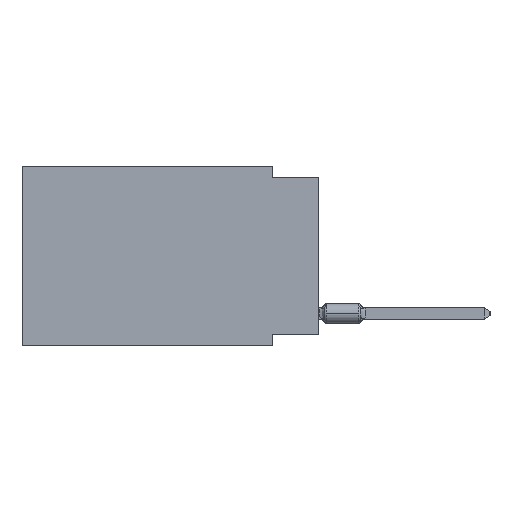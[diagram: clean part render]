
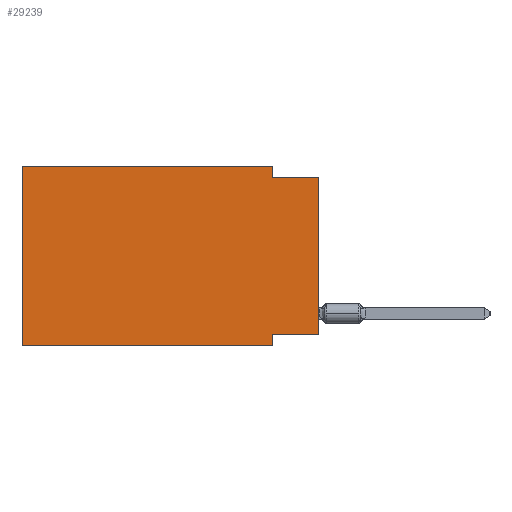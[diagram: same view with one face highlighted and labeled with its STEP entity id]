
A CAD part, left-side view. The second image highlights one B-rep face of the part: STEP entity #29239.
In plain terms, the highlighted planar face has unit normal (-1, 0, 0).
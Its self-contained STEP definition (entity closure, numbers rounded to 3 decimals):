
#490 = VECTOR ( 'NONE', #22707, 1000. ) ;
#543 = DIRECTION ( 'NONE',  ( 0., 0., 1. ) ) ;
#1589 = ORIENTED_EDGE ( 'NONE', *, *, #5395, .T. ) ;
#1787 = LINE ( 'NONE', #32065, #10415 ) ;
#1984 = CARTESIAN_POINT ( 'NONE',  ( 0., 0., -0.635 ) ) ;
#2835 = CARTESIAN_POINT ( 'NONE',  ( 0., 2.54, 0. ) ) ;
#3249 = CARTESIAN_POINT ( 'NONE',  ( 0., 2.54, -9.906 ) ) ;
#4704 = DIRECTION ( 'NONE',  ( 0., -1., 0. ) ) ;
#5305 = CARTESIAN_POINT ( 'NONE',  ( 0., 16.383, 0. ) ) ;
#5395 = EDGE_CURVE ( 'NONE', #22550, #21201, #22999, .T. ) ;
#6250 = LINE ( 'NONE', #11909, #23976 ) ;
#6570 = CARTESIAN_POINT ( 'NONE',  ( 0., 2.54, -9.906 ) ) ;
#6589 = VECTOR ( 'NONE', #13106, 1000. ) ;
#8101 = AXIS2_PLACEMENT_3D ( 'NONE', #5305, #10420, #24469 ) ;
#8115 = DIRECTION ( 'NONE',  ( 0., 1., 0. ) ) ;
#8686 = VERTEX_POINT ( 'NONE', #35474 ) ;
#9042 = VERTEX_POINT ( 'NONE', #18314 ) ;
#10415 = VECTOR ( 'NONE', #4704, 1000. ) ;
#10420 = DIRECTION ( 'NONE',  ( 1., 0., 0. ) ) ;
#10931 = EDGE_LOOP ( 'NONE', ( #1589, #17435, #23815, #11695, #15495, #32703, #25203, #31694 ) ) ;
#11402 = LINE ( 'NONE', #2835, #490 ) ;
#11695 = ORIENTED_EDGE ( 'NONE', *, *, #28238, .F. ) ;
#11909 = CARTESIAN_POINT ( 'NONE',  ( 0., 16.383, -9.906 ) ) ;
#12170 = VECTOR ( 'NONE', #8115, 1000. ) ;
#13106 = DIRECTION ( 'NONE',  ( 0., -1., 0. ) ) ;
#13522 = FACE_OUTER_BOUND ( 'NONE', #10931, .T. ) ;
#13954 = LINE ( 'NONE', #19438, #12170 ) ;
#14029 = EDGE_CURVE ( 'NONE', #22843, #21201, #26985, .T. ) ;
#15120 = VECTOR ( 'NONE', #26096, 1000. ) ;
#15495 = ORIENTED_EDGE ( 'NONE', *, *, #29360, .F. ) ;
#17435 = ORIENTED_EDGE ( 'NONE', *, *, #14029, .F. ) ;
#17524 = LINE ( 'NONE', #22629, #34335 ) ;
#17923 = VERTEX_POINT ( 'NONE', #29832 ) ;
#18314 = CARTESIAN_POINT ( 'NONE',  ( 0., 16.383, -9.906 ) ) ;
#19177 = PLANE ( 'NONE',  #8101 ) ;
#19239 = CARTESIAN_POINT ( 'NONE',  ( 0., 2.54, -0.635 ) ) ;
#19438 = CARTESIAN_POINT ( 'NONE',  ( 0., 0., -9.271 ) ) ;
#20259 = DIRECTION ( 'NONE',  ( 0., 0., 1. ) ) ;
#20760 = EDGE_CURVE ( 'NONE', #22550, #8686, #13954, .T. ) ;
#21201 = VERTEX_POINT ( 'NONE', #29580 ) ;
#22550 = VERTEX_POINT ( 'NONE', #30856 ) ;
#22629 = CARTESIAN_POINT ( 'NONE',  ( 0., 16.383, 0. ) ) ;
#22706 = VERTEX_POINT ( 'NONE', #26917 ) ;
#22707 = DIRECTION ( 'NONE',  ( 0., 0., -1. ) ) ;
#22843 = VERTEX_POINT ( 'NONE', #19239 ) ;
#22999 = LINE ( 'NONE', #34123, #31280 ) ;
#23815 = ORIENTED_EDGE ( 'NONE', *, *, #34801, .F. ) ;
#23852 = EDGE_CURVE ( 'NONE', #9042, #31517, #6250, .T. ) ;
#23976 = VECTOR ( 'NONE', #29406, 1000. ) ;
#24469 = DIRECTION ( 'NONE',  ( 0., 0., -1. ) ) ;
#25203 = ORIENTED_EDGE ( 'NONE', *, *, #28437, .F. ) ;
#26096 = DIRECTION ( 'NONE',  ( 0., 0., -1. ) ) ;
#26917 = CARTESIAN_POINT ( 'NONE',  ( 0., 2.54, 0. ) ) ;
#26985 = LINE ( 'NONE', #1984, #6589 ) ;
#28238 = EDGE_CURVE ( 'NONE', #17923, #22706, #1787, .T. ) ;
#28437 = EDGE_CURVE ( 'NONE', #8686, #31517, #28453, .T. ) ;
#28453 = LINE ( 'NONE', #6570, #15120 ) ;
#29239 = ADVANCED_FACE ( 'NONE', ( #13522 ), #19177, .F. ) ;
#29360 = EDGE_CURVE ( 'NONE', #9042, #17923, #17524, .T. ) ;
#29406 = DIRECTION ( 'NONE',  ( 0., -1., 0. ) ) ;
#29580 = CARTESIAN_POINT ( 'NONE',  ( 0., 0., -0.635 ) ) ;
#29832 = CARTESIAN_POINT ( 'NONE',  ( 0., 16.383, 0. ) ) ;
#30856 = CARTESIAN_POINT ( 'NONE',  ( 0., 0., -9.271 ) ) ;
#31280 = VECTOR ( 'NONE', #20259, 1000. ) ;
#31517 = VERTEX_POINT ( 'NONE', #3249 ) ;
#31694 = ORIENTED_EDGE ( 'NONE', *, *, #20760, .F. ) ;
#32065 = CARTESIAN_POINT ( 'NONE',  ( 0., 16.383, 0. ) ) ;
#32703 = ORIENTED_EDGE ( 'NONE', *, *, #23852, .T. ) ;
#34123 = CARTESIAN_POINT ( 'NONE',  ( 0., 0., 0. ) ) ;
#34335 = VECTOR ( 'NONE', #543, 1000. ) ;
#34801 = EDGE_CURVE ( 'NONE', #22706, #22843, #11402, .T. ) ;
#35474 = CARTESIAN_POINT ( 'NONE',  ( 0., 2.54, -9.271 ) ) ;
